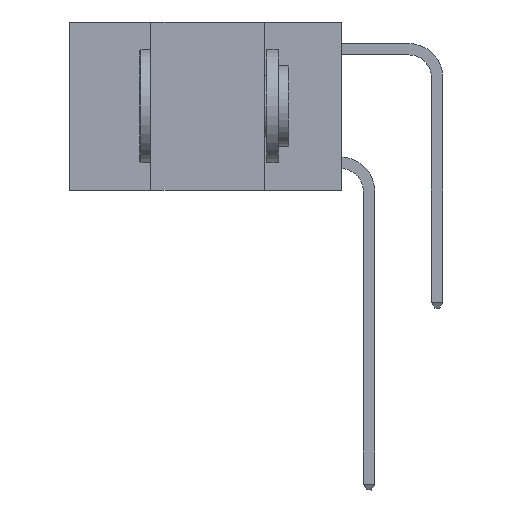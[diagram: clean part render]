
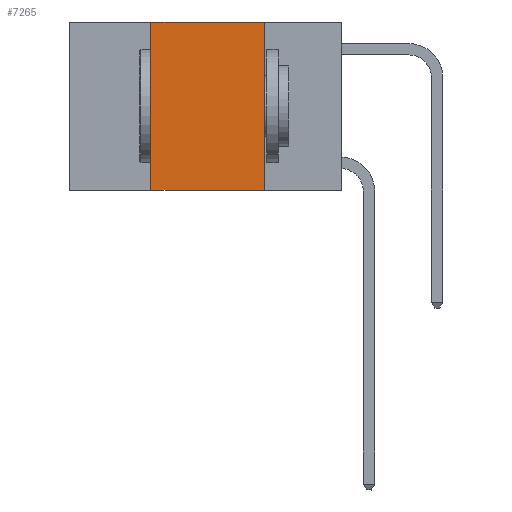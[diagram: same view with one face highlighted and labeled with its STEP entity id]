
A CAD part, left-side view. The second image highlights one B-rep face of the part: STEP entity #7265.
In plain terms, the highlighted planar face has unit normal (-1, 0, 0).
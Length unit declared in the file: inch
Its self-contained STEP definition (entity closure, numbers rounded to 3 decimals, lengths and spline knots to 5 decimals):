
#164 = VECTOR ( 'NONE', #12895, 39.37008 ) ;
#2025 = CARTESIAN_POINT ( 'NONE',  ( 0., 0.6, 0. ) ) ;
#2645 = CARTESIAN_POINT ( 'NONE',  ( 0., 0.6, 0. ) ) ;
#3163 = VERTEX_POINT ( 'NONE', #17113 ) ;
#3385 = VECTOR ( 'NONE', #14384, 39.37008 ) ;
#4406 = ORIENTED_EDGE ( 'NONE', *, *, #7094, .F. ) ;
#4804 = VECTOR ( 'NONE', #9178, 39.37008 ) ;
#5094 = VERTEX_POINT ( 'NONE', #25207 ) ;
#5912 = CARTESIAN_POINT ( 'NONE',  ( 0., 0.17, -0.37 ) ) ;
#6536 = CARTESIAN_POINT ( 'NONE',  ( 0., 0.17, 0. ) ) ;
#6750 = CARTESIAN_POINT ( 'NONE',  ( 0., 0.6, -0.37 ) ) ;
#7094 = EDGE_CURVE ( 'NONE', #17926, #3163, #13240, .T. ) ;
#7265 = ADVANCED_FACE ( 'NONE', ( #21592 ), #10012, .F. ) ;
#7945 = CARTESIAN_POINT ( 'NONE',  ( 0., 0.42, 0. ) ) ;
#8882 = EDGE_CURVE ( 'NONE', #5094, #25137, #15431, .T. ) ;
#9178 = DIRECTION ( 'NONE',  ( 0., -1., 0. ) ) ;
#10012 = PLANE ( 'NONE',  #23630 ) ;
#10521 = EDGE_CURVE ( 'NONE', #3163, #5094, #22878, .T. ) ;
#12529 = DIRECTION ( 'NONE',  ( 1., 0., 0. ) ) ;
#12895 = DIRECTION ( 'NONE',  ( 0., 0., 1. ) ) ;
#13240 = LINE ( 'NONE', #7945, #164 ) ;
#14384 = DIRECTION ( 'NONE',  ( 0., -1., 0. ) ) ;
#15431 = LINE ( 'NONE', #6536, #28285 ) ;
#17113 = CARTESIAN_POINT ( 'NONE',  ( 0., 0.42, 0. ) ) ;
#17848 = LINE ( 'NONE', #6750, #4804 ) ;
#17926 = VERTEX_POINT ( 'NONE', #26113 ) ;
#21592 = FACE_OUTER_BOUND ( 'NONE', #27332, .T. ) ;
#22878 = LINE ( 'NONE', #2025, #3385 ) ;
#23572 = DIRECTION ( 'NONE',  ( 0., 0., -1. ) ) ;
#23630 = AXIS2_PLACEMENT_3D ( 'NONE', #2645, #12529, #29512 ) ;
#25137 = VERTEX_POINT ( 'NONE', #5912 ) ;
#25207 = CARTESIAN_POINT ( 'NONE',  ( 0., 0.17, 0. ) ) ;
#26113 = CARTESIAN_POINT ( 'NONE',  ( 0., 0.42, -0.37 ) ) ;
#27332 = EDGE_LOOP ( 'NONE', ( #28030, #28801, #4406, #27408 ) ) ;
#27408 = ORIENTED_EDGE ( 'NONE', *, *, #29624, .T. ) ;
#28030 = ORIENTED_EDGE ( 'NONE', *, *, #8882, .F. ) ;
#28285 = VECTOR ( 'NONE', #23572, 39.37008 ) ;
#28801 = ORIENTED_EDGE ( 'NONE', *, *, #10521, .F. ) ;
#29512 = DIRECTION ( 'NONE',  ( 0., 0., -1. ) ) ;
#29624 = EDGE_CURVE ( 'NONE', #17926, #25137, #17848, .T. ) ;
